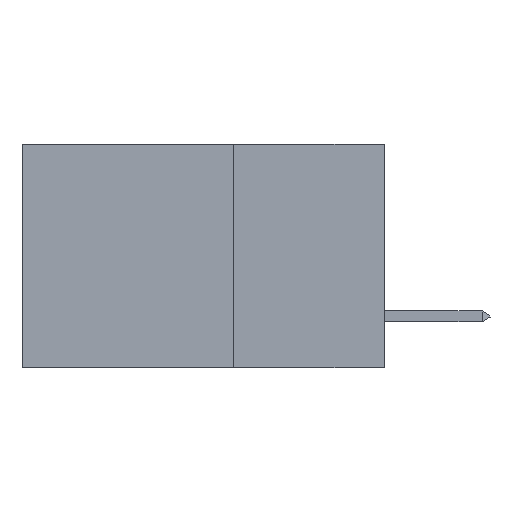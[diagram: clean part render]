
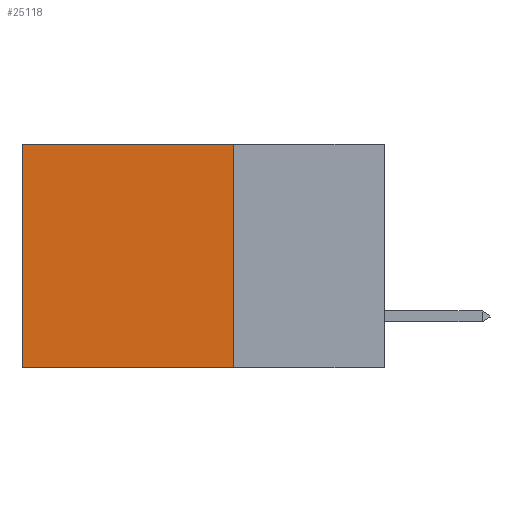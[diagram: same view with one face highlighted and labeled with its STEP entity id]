
A CAD part, left-side view. The second image highlights one B-rep face of the part: STEP entity #25118.
In plain terms, the highlighted planar face has unit normal (-1, 0, 0).
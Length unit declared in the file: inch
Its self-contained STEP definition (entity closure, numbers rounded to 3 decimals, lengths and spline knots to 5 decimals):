
#726 = DIRECTION ( 'NONE',  ( 0., 1., 0. ) ) ;
#902 = CARTESIAN_POINT ( 'NONE',  ( 0.2875, 0.25, -0.37 ) ) ;
#1659 = ORIENTED_EDGE ( 'NONE', *, *, #15694, .F. ) ;
#2220 = EDGE_LOOP ( 'NONE', ( #11516, #1659, #5048, #6039 ) ) ;
#2891 = EDGE_CURVE ( 'NONE', #6134, #15571, #14285, .T. ) ;
#3155 = VERTEX_POINT ( 'NONE', #20528 ) ;
#4072 = LINE ( 'NONE', #12095, #25537 ) ;
#5048 = ORIENTED_EDGE ( 'NONE', *, *, #12452, .F. ) ;
#5133 = LINE ( 'NONE', #902, #15265 ) ;
#6039 = ORIENTED_EDGE ( 'NONE', *, *, #9723, .T. ) ;
#6134 = VERTEX_POINT ( 'NONE', #21980 ) ;
#6286 = DIRECTION ( 'NONE',  ( 0., 0., -1. ) ) ;
#9168 = DIRECTION ( 'NONE',  ( 0., 0., -1. ) ) ;
#9578 = VERTEX_POINT ( 'NONE', #25420 ) ;
#9723 = EDGE_CURVE ( 'NONE', #3155, #6134, #4072, .T. ) ;
#10828 = VECTOR ( 'NONE', #6286, 39.37008 ) ;
#11516 = ORIENTED_EDGE ( 'NONE', *, *, #2891, .T. ) ;
#12095 = CARTESIAN_POINT ( 'NONE',  ( 0.2875, 0.25, 0. ) ) ;
#12452 = EDGE_CURVE ( 'NONE', #3155, #9578, #25812, .T. ) ;
#13345 = PLANE ( 'NONE',  #20072 ) ;
#14285 = LINE ( 'NONE', #22261, #10828 ) ;
#15265 = VECTOR ( 'NONE', #726, 39.37008 ) ;
#15571 = VERTEX_POINT ( 'NONE', #24363 ) ;
#15694 = EDGE_CURVE ( 'NONE', #9578, #15571, #5133, .T. ) ;
#19155 = CARTESIAN_POINT ( 'NONE',  ( 0.2875, 0.25, 0. ) ) ;
#20072 = AXIS2_PLACEMENT_3D ( 'NONE', #25492, #25756, #23403 ) ;
#20528 = CARTESIAN_POINT ( 'NONE',  ( 0.2875, 0.25, 0. ) ) ;
#21067 = VECTOR ( 'NONE', #9168, 39.37008 ) ;
#21980 = CARTESIAN_POINT ( 'NONE',  ( 0.2875, 0.6, 0. ) ) ;
#22261 = CARTESIAN_POINT ( 'NONE',  ( 0.2875, 0.6, 0. ) ) ;
#22741 = FACE_OUTER_BOUND ( 'NONE', #2220, .T. ) ;
#23403 = DIRECTION ( 'NONE',  ( 0., 0., -1. ) ) ;
#24086 = DIRECTION ( 'NONE',  ( 0., 1., 0. ) ) ;
#24363 = CARTESIAN_POINT ( 'NONE',  ( 0.2875, 0.6, -0.37 ) ) ;
#25118 = ADVANCED_FACE ( 'NONE', ( #22741 ), #13345, .F. ) ;
#25420 = CARTESIAN_POINT ( 'NONE',  ( 0.2875, 0.25, -0.37 ) ) ;
#25492 = CARTESIAN_POINT ( 'NONE',  ( 0.2875, 0.25, 0. ) ) ;
#25537 = VECTOR ( 'NONE', #24086, 39.37008 ) ;
#25756 = DIRECTION ( 'NONE',  ( 1., 0., 0. ) ) ;
#25812 = LINE ( 'NONE', #19155, #21067 ) ;
